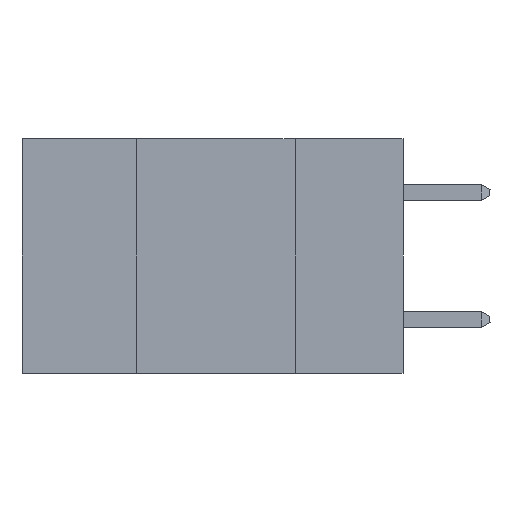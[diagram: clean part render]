
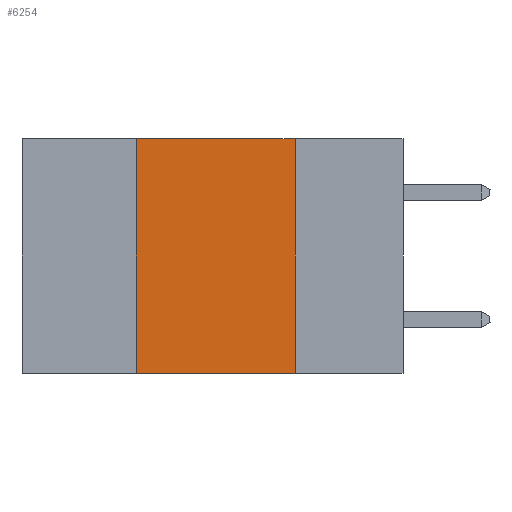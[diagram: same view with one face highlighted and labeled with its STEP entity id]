
A CAD part, left-side view. The second image highlights one B-rep face of the part: STEP entity #6254.
In plain terms, the highlighted planar face has unit normal (-1, 0, 0).
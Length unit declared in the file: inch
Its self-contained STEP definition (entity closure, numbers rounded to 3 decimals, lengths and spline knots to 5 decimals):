
#604 = VECTOR ( 'NONE', #3394, 39.37008 ) ;
#1078 = ORIENTED_EDGE ( 'NONE', *, *, #25935, .F. ) ;
#2366 = ORIENTED_EDGE ( 'NONE', *, *, #13620, .F. ) ;
#2420 = DIRECTION ( 'NONE',  ( 0., 0., 1. ) ) ;
#3126 = LINE ( 'NONE', #21886, #25649 ) ;
#3165 = AXIS2_PLACEMENT_3D ( 'NONE', #22980, #20812, #27610 ) ;
#3394 = DIRECTION ( 'NONE',  ( 0., -1., 0. ) ) ;
#5106 = CARTESIAN_POINT ( 'NONE',  ( 0., 0.6, -0.37 ) ) ;
#5848 = CARTESIAN_POINT ( 'NONE',  ( 0., 0.17, 0. ) ) ;
#6254 = ADVANCED_FACE ( 'NONE', ( #13997 ), #7086, .F. ) ;
#7086 = PLANE ( 'NONE',  #3165 ) ;
#7242 = EDGE_LOOP ( 'NONE', ( #18088, #1078, #2366, #17526 ) ) ;
#8061 = LINE ( 'NONE', #23430, #21729 ) ;
#8482 = EDGE_CURVE ( 'NONE', #25513, #20646, #10817, .T. ) ;
#9783 = CARTESIAN_POINT ( 'NONE',  ( 0., 0.6, 0. ) ) ;
#10148 = LINE ( 'NONE', #9783, #604 ) ;
#10817 = LINE ( 'NONE', #5106, #27314 ) ;
#10844 = VERTEX_POINT ( 'NONE', #24086 ) ;
#13620 = EDGE_CURVE ( 'NONE', #25513, #10844, #8061, .T. ) ;
#13997 = FACE_OUTER_BOUND ( 'NONE', #7242, .T. ) ;
#15051 = VERTEX_POINT ( 'NONE', #5848 ) ;
#17526 = ORIENTED_EDGE ( 'NONE', *, *, #8482, .T. ) ;
#18088 = ORIENTED_EDGE ( 'NONE', *, *, #27650, .F. ) ;
#19462 = DIRECTION ( 'NONE',  ( 0., 0., -1. ) ) ;
#19691 = CARTESIAN_POINT ( 'NONE',  ( 0., 0.42, -0.37 ) ) ;
#19753 = CARTESIAN_POINT ( 'NONE',  ( 0., 0.17, -0.37 ) ) ;
#20646 = VERTEX_POINT ( 'NONE', #19753 ) ;
#20812 = DIRECTION ( 'NONE',  ( 1., 0., 0. ) ) ;
#21532 = DIRECTION ( 'NONE',  ( 0., -1., 0. ) ) ;
#21729 = VECTOR ( 'NONE', #2420, 39.37008 ) ;
#21886 = CARTESIAN_POINT ( 'NONE',  ( 0., 0.17, 0. ) ) ;
#22980 = CARTESIAN_POINT ( 'NONE',  ( 0., 0.6, 0. ) ) ;
#23430 = CARTESIAN_POINT ( 'NONE',  ( 0., 0.42, 0. ) ) ;
#24086 = CARTESIAN_POINT ( 'NONE',  ( 0., 0.42, 0. ) ) ;
#25513 = VERTEX_POINT ( 'NONE', #19691 ) ;
#25649 = VECTOR ( 'NONE', #19462, 39.37008 ) ;
#25935 = EDGE_CURVE ( 'NONE', #10844, #15051, #10148, .T. ) ;
#27314 = VECTOR ( 'NONE', #21532, 39.37008 ) ;
#27610 = DIRECTION ( 'NONE',  ( 0., 0., -1. ) ) ;
#27650 = EDGE_CURVE ( 'NONE', #15051, #20646, #3126, .T. ) ;
